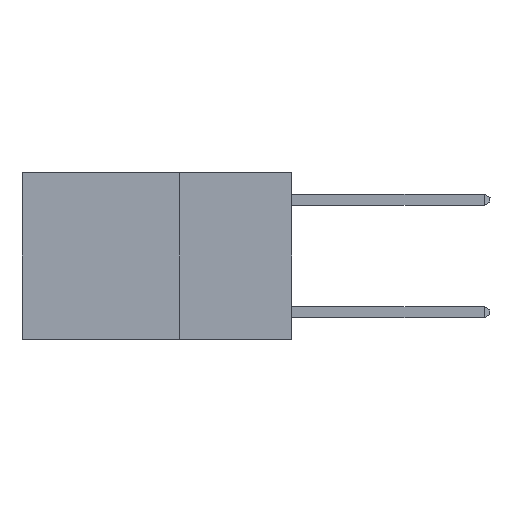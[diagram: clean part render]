
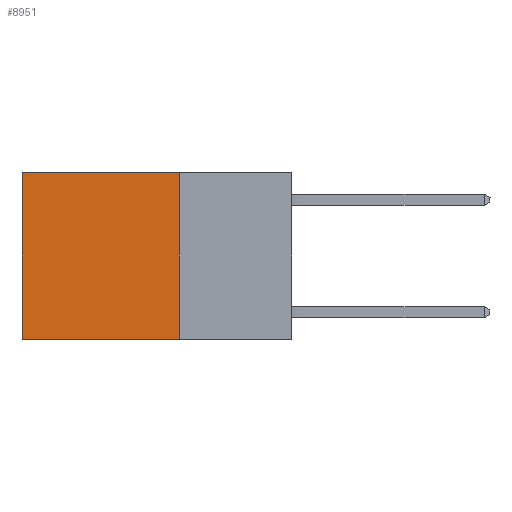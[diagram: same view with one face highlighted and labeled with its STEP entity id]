
A CAD part, left-side view. The second image highlights one B-rep face of the part: STEP entity #8951.
In plain terms, the highlighted planar face has unit normal (-1, 0, 0).
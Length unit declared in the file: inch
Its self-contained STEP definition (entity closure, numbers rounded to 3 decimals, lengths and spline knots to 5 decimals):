
#793 = DIRECTION ( 'NONE',  ( 0., 1., 0. ) ) ;
#1121 = CARTESIAN_POINT ( 'NONE',  ( 0.2625, 0.25, 0. ) ) ;
#1173 = VECTOR ( 'NONE', #7289, 39.37008 ) ;
#1179 = CARTESIAN_POINT ( 'NONE',  ( 0.2625, 0.6, -0.37 ) ) ;
#1609 = LINE ( 'NONE', #3661, #1173 ) ;
#1718 = CARTESIAN_POINT ( 'NONE',  ( 0.2625, 0.6, 0. ) ) ;
#1931 = VERTEX_POINT ( 'NONE', #6986 ) ;
#2139 = VECTOR ( 'NONE', #793, 39.37008 ) ;
#2519 = ORIENTED_EDGE ( 'NONE', *, *, #6418, .F. ) ;
#2659 = DIRECTION ( 'NONE',  ( 0., 0., -1. ) ) ;
#3122 = DIRECTION ( 'NONE',  ( 1., 0., 0. ) ) ;
#3173 = ORIENTED_EDGE ( 'NONE', *, *, #5149, .T. ) ;
#3258 = ORIENTED_EDGE ( 'NONE', *, *, #9034, .F. ) ;
#3661 = CARTESIAN_POINT ( 'NONE',  ( 0.2625, 0.25, -0.37 ) ) ;
#3969 = ORIENTED_EDGE ( 'NONE', *, *, #6807, .T. ) ;
#4041 = CARTESIAN_POINT ( 'NONE',  ( 0.2625, 0.25, -0.37 ) ) ;
#4737 = EDGE_LOOP ( 'NONE', ( #3969, #3258, #2519, #3173 ) ) ;
#5069 = FACE_OUTER_BOUND ( 'NONE', #4737, .T. ) ;
#5149 = EDGE_CURVE ( 'NONE', #6961, #1931, #6501, .T. ) ;
#5743 = VECTOR ( 'NONE', #11456, 39.37008 ) ;
#6002 = DIRECTION ( 'NONE',  ( 0., 0., -1. ) ) ;
#6418 = EDGE_CURVE ( 'NONE', #6961, #10668, #12269, .T. ) ;
#6501 = LINE ( 'NONE', #6629, #2139 ) ;
#6629 = CARTESIAN_POINT ( 'NONE',  ( 0.2625, 0.25, 0. ) ) ;
#6807 = EDGE_CURVE ( 'NONE', #1931, #8085, #7411, .T. ) ;
#6961 = VERTEX_POINT ( 'NONE', #8530 ) ;
#6986 = CARTESIAN_POINT ( 'NONE',  ( 0.2625, 0.6, 0. ) ) ;
#7289 = DIRECTION ( 'NONE',  ( 0., 1., 0. ) ) ;
#7411 = LINE ( 'NONE', #1718, #11923 ) ;
#8085 = VERTEX_POINT ( 'NONE', #1179 ) ;
#8530 = CARTESIAN_POINT ( 'NONE',  ( 0.2625, 0.25, 0. ) ) ;
#8951 = ADVANCED_FACE ( 'NONE', ( #5069 ), #11658, .F. ) ;
#9034 = EDGE_CURVE ( 'NONE', #10668, #8085, #1609, .T. ) ;
#9549 = CARTESIAN_POINT ( 'NONE',  ( 0.2625, 0.25, 0. ) ) ;
#9966 = AXIS2_PLACEMENT_3D ( 'NONE', #1121, #3122, #6002 ) ;
#10668 = VERTEX_POINT ( 'NONE', #4041 ) ;
#11456 = DIRECTION ( 'NONE',  ( 0., 0., -1. ) ) ;
#11658 = PLANE ( 'NONE',  #9966 ) ;
#11923 = VECTOR ( 'NONE', #2659, 39.37008 ) ;
#12269 = LINE ( 'NONE', #9549, #5743 ) ;
